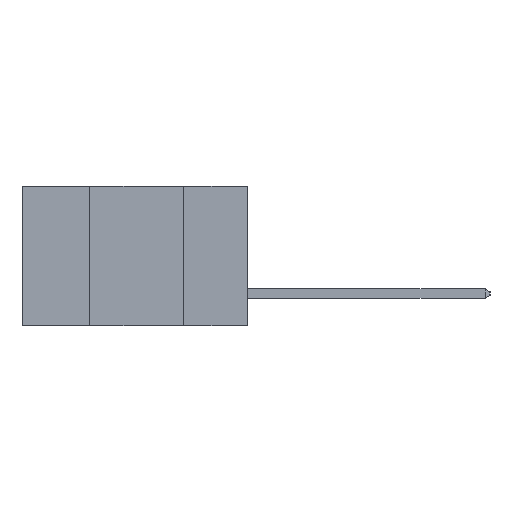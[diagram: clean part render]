
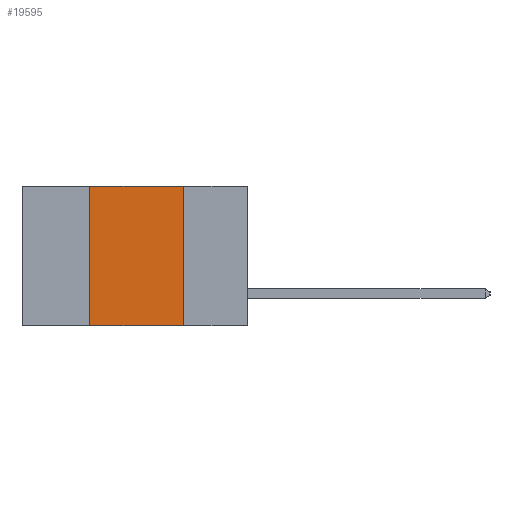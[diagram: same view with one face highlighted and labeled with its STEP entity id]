
A CAD part, left-side view. The second image highlights one B-rep face of the part: STEP entity #19595.
In plain terms, the highlighted planar face has unit normal (-1, 0, 0).
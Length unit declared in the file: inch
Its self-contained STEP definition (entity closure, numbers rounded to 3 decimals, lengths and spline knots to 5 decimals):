
#404 = EDGE_CURVE ( 'NONE', #10962, #15481, #16096, .T. ) ;
#690 = DIRECTION ( 'NONE',  ( 0., 0., -1. ) ) ;
#1371 = VERTEX_POINT ( 'NONE', #12669 ) ;
#1646 = LINE ( 'NONE', #21802, #15935 ) ;
#2860 = DIRECTION ( 'NONE',  ( 0., 0., -1. ) ) ;
#5222 = AXIS2_PLACEMENT_3D ( 'NONE', #17659, #14042, #2860 ) ;
#5305 = VECTOR ( 'NONE', #690, 39.37008 ) ;
#7556 = VERTEX_POINT ( 'NONE', #23559 ) ;
#7720 = ORIENTED_EDGE ( 'NONE', *, *, #15766, .F. ) ;
#7799 = EDGE_CURVE ( 'NONE', #7556, #1371, #12717, .T. ) ;
#7891 = CARTESIAN_POINT ( 'NONE',  ( 0., 0.6, 0. ) ) ;
#8511 = ORIENTED_EDGE ( 'NONE', *, *, #404, .F. ) ;
#8803 = ORIENTED_EDGE ( 'NONE', *, *, #23089, .F. ) ;
#9751 = ORIENTED_EDGE ( 'NONE', *, *, #7799, .T. ) ;
#10013 = DIRECTION ( 'NONE',  ( 0., -1., 0. ) ) ;
#10226 = PLANE ( 'NONE',  #5222 ) ;
#10273 = LINE ( 'NONE', #21033, #5305 ) ;
#10882 = FACE_OUTER_BOUND ( 'NONE', #12159, .T. ) ;
#10962 = VERTEX_POINT ( 'NONE', #18659 ) ;
#11128 = VECTOR ( 'NONE', #13889, 39.37008 ) ;
#12159 = EDGE_LOOP ( 'NONE', ( #7720, #8511, #8803, #9751 ) ) ;
#12631 = DIRECTION ( 'NONE',  ( 0., 0., 1. ) ) ;
#12669 = CARTESIAN_POINT ( 'NONE',  ( 0., 0.17, -0.37 ) ) ;
#12717 = LINE ( 'NONE', #20123, #17627 ) ;
#12929 = CARTESIAN_POINT ( 'NONE',  ( 0., 0.17, 0. ) ) ;
#13889 = DIRECTION ( 'NONE',  ( 0., -1., 0. ) ) ;
#14042 = DIRECTION ( 'NONE',  ( 1., 0., 0. ) ) ;
#15481 = VERTEX_POINT ( 'NONE', #12929 ) ;
#15766 = EDGE_CURVE ( 'NONE', #15481, #1371, #10273, .T. ) ;
#15935 = VECTOR ( 'NONE', #12631, 39.37008 ) ;
#16096 = LINE ( 'NONE', #7891, #11128 ) ;
#17627 = VECTOR ( 'NONE', #10013, 39.37008 ) ;
#17659 = CARTESIAN_POINT ( 'NONE',  ( 0., 0.6, 0. ) ) ;
#18659 = CARTESIAN_POINT ( 'NONE',  ( 0., 0.42, 0. ) ) ;
#19595 = ADVANCED_FACE ( 'NONE', ( #10882 ), #10226, .F. ) ;
#20123 = CARTESIAN_POINT ( 'NONE',  ( 0., 0.6, -0.37 ) ) ;
#21033 = CARTESIAN_POINT ( 'NONE',  ( 0., 0.17, 0. ) ) ;
#21802 = CARTESIAN_POINT ( 'NONE',  ( 0., 0.42, 0. ) ) ;
#23089 = EDGE_CURVE ( 'NONE', #7556, #10962, #1646, .T. ) ;
#23559 = CARTESIAN_POINT ( 'NONE',  ( 0., 0.42, -0.37 ) ) ;
